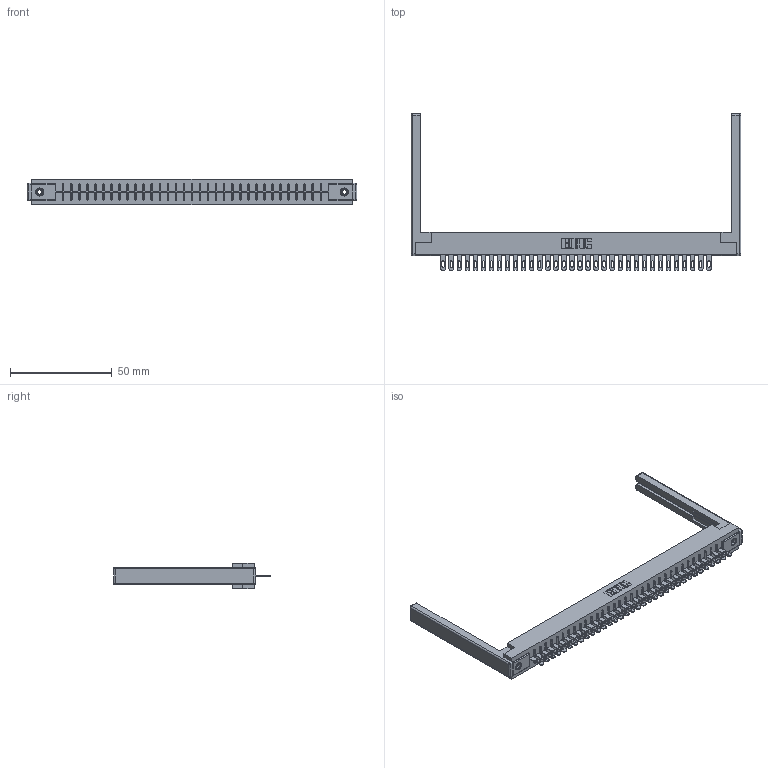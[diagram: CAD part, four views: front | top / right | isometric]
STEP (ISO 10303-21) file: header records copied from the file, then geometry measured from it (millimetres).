
FILE_DESCRIPTION (( 'STEP AP203' ), '1' );
FILE_NAME ('356-034-400-168.STEP', '2020-09-23T21:57:34', ( '' ), ( '' ), 'SwSTEP 2.0', 'SolidWorks 2020', '' );
FILE_SCHEMA (( 'CONFIG_CONTROL_DESIGN' ));
Length unit declared in the file: inch
Products named in the file (5): 307-220-068; 356-034-400-168; 306 Part_.156 Dia; 345-250-001_345-250-001-102; 306-290-001_100
Assembly tree (39 placements, depth 2):
  356-034-400-168
    306 Part_.156 Dia
    306-290-001_100  x34
    345-250-001_345-250-001-102  x2
    307-220-068  x2
Bounding box: 162.15 x 77.17 x 12.7 mm (x, y, z)
Volume: 22328.7 mm3; surface area: 23016.7 mm2
Topology: 39 solids, 39 shells, 2854 faces, 8016 edges, 5140 vertices
Faces by surface type: plane 1856, cylinder 838, sphere 144, cone 12, torus 4
Entity records: 35666 total; most frequent: CARTESIAN_POINT 5954, ORIENTED_EDGE 5894, DIRECTION 5885, EDGE_CURVE 2947, VECTOR 2295, LINE 2295, VERTEX_POINT 1864, AXIS2_PLACEMENT_3D 1795
